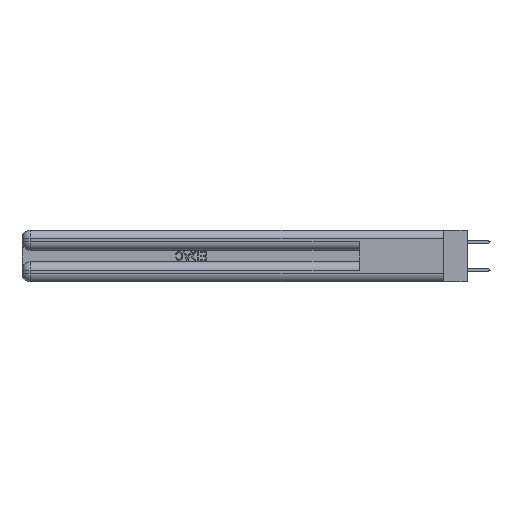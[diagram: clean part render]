
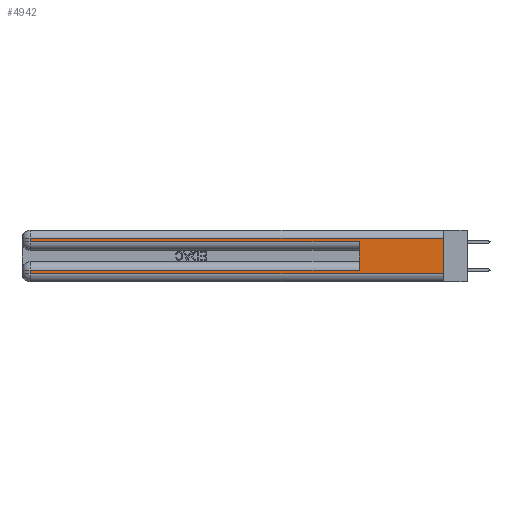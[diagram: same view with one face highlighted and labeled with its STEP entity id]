
A CAD part, left-side view. The second image highlights one B-rep face of the part: STEP entity #4942.
In plain terms, the highlighted planar face has unit normal (-1, 0, 0).
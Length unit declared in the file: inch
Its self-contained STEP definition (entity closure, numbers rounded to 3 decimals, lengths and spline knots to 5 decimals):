
#1281 = LINE ( 'NONE', #5672, #41660 ) ;
#2122 = CARTESIAN_POINT ( 'NONE',  ( 0., 0., 0.06 ) ) ;
#2264 = ORIENTED_EDGE ( 'NONE', *, *, #47043, .T. ) ;
#3876 = EDGE_LOOP ( 'NONE', ( #27338, #7959, #11782, #43535, #30593, #14664, #40190, #2264 ) ) ;
#4942 = ADVANCED_FACE ( 'NONE', ( #32410 ), #41638, .F. ) ;
#4976 = CARTESIAN_POINT ( 'NONE',  ( 0., 0., 0.31 ) ) ;
#5428 = VECTOR ( 'NONE', #43434, 39.37008 ) ;
#5592 = EDGE_CURVE ( 'NONE', #45847, #29594, #26237, .T. ) ;
#5672 = CARTESIAN_POINT ( 'NONE',  ( 0., 0.6, 0.145 ) ) ;
#6160 = DIRECTION ( 'NONE',  ( 0., 0., -1. ) ) ;
#7959 = ORIENTED_EDGE ( 'NONE', *, *, #23020, .T. ) ;
#8643 = VERTEX_POINT ( 'NONE', #48843 ) ;
#8798 = LINE ( 'NONE', #22082, #27135 ) ;
#9466 = DIRECTION ( 'NONE',  ( 0., 0., 1. ) ) ;
#9813 = DIRECTION ( 'NONE',  ( 0., -1., 0. ) ) ;
#11782 = ORIENTED_EDGE ( 'NONE', *, *, #45317, .T. ) ;
#12026 = LINE ( 'NONE', #26265, #30928 ) ;
#14664 = ORIENTED_EDGE ( 'NONE', *, *, #50376, .T. ) ;
#15242 = CARTESIAN_POINT ( 'NONE',  ( 0., 2.94, 0.285 ) ) ;
#16921 = DIRECTION ( 'NONE',  ( 0., 1., 0. ) ) ;
#18801 = EDGE_CURVE ( 'NONE', #29335, #29594, #1281, .T. ) ;
#19373 = VERTEX_POINT ( 'NONE', #39662 ) ;
#19379 = LINE ( 'NONE', #39591, #37740 ) ;
#19396 = DIRECTION ( 'NONE',  ( 0., 0., -1. ) ) ;
#20255 = DIRECTION ( 'NONE',  ( 0., 0., -1. ) ) ;
#21742 = VERTEX_POINT ( 'NONE', #41632 ) ;
#21830 = VECTOR ( 'NONE', #9813, 39.37008 ) ;
#22082 = CARTESIAN_POINT ( 'NONE',  ( 0., 0., 0.37 ) ) ;
#22130 = VERTEX_POINT ( 'NONE', #4976 ) ;
#22729 = CARTESIAN_POINT ( 'NONE',  ( 0., 2.94, 0.37 ) ) ;
#23020 = EDGE_CURVE ( 'NONE', #22130, #42569, #12026, .T. ) ;
#23848 = CARTESIAN_POINT ( 'NONE',  ( 0., 0., 0.37 ) ) ;
#26237 = LINE ( 'NONE', #27685, #5428 ) ;
#26265 = CARTESIAN_POINT ( 'NONE',  ( 0., 0., 0.31 ) ) ;
#26968 = LINE ( 'NONE', #40497, #33716 ) ;
#27076 = DIRECTION ( 'NONE',  ( 1., 0., 0. ) ) ;
#27135 = VECTOR ( 'NONE', #6160, 39.37008 ) ;
#27338 = ORIENTED_EDGE ( 'NONE', *, *, #29759, .F. ) ;
#27685 = CARTESIAN_POINT ( 'NONE',  ( 0., 0., 0.285 ) ) ;
#27855 = LINE ( 'NONE', #22729, #42546 ) ;
#28036 = EDGE_CURVE ( 'NONE', #19373, #21742, #27855, .T. ) ;
#29335 = VERTEX_POINT ( 'NONE', #47261 ) ;
#29594 = VERTEX_POINT ( 'NONE', #44347 ) ;
#29759 = EDGE_CURVE ( 'NONE', #22130, #8643, #8798, .T. ) ;
#30347 = DIRECTION ( 'NONE',  ( 0., 1., 0. ) ) ;
#30593 = ORIENTED_EDGE ( 'NONE', *, *, #18801, .F. ) ;
#30928 = VECTOR ( 'NONE', #30347, 39.37008 ) ;
#32154 = CARTESIAN_POINT ( 'NONE',  ( 0., 2.94, 0.31 ) ) ;
#32410 = FACE_OUTER_BOUND ( 'NONE', #3876, .T. ) ;
#33716 = VECTOR ( 'NONE', #16921, 39.37008 ) ;
#37740 = VECTOR ( 'NONE', #20255, 39.37008 ) ;
#39551 = LINE ( 'NONE', #2122, #21830 ) ;
#39591 = CARTESIAN_POINT ( 'NONE',  ( 0., 2.94, 0.37 ) ) ;
#39662 = CARTESIAN_POINT ( 'NONE',  ( 0., 2.94, 0.085 ) ) ;
#40190 = ORIENTED_EDGE ( 'NONE', *, *, #28036, .T. ) ;
#40497 = CARTESIAN_POINT ( 'NONE',  ( 0., 0., 0.085 ) ) ;
#41632 = CARTESIAN_POINT ( 'NONE',  ( 0., 2.94, 0.06 ) ) ;
#41638 = PLANE ( 'NONE',  #46428 ) ;
#41660 = VECTOR ( 'NONE', #9466, 39.37008 ) ;
#41914 = DIRECTION ( 'NONE',  ( 0., 0., -1. ) ) ;
#42546 = VECTOR ( 'NONE', #41914, 39.37008 ) ;
#42569 = VERTEX_POINT ( 'NONE', #32154 ) ;
#43434 = DIRECTION ( 'NONE',  ( 0., -1., 0. ) ) ;
#43535 = ORIENTED_EDGE ( 'NONE', *, *, #5592, .T. ) ;
#44347 = CARTESIAN_POINT ( 'NONE',  ( 0., 0.6, 0.285 ) ) ;
#45317 = EDGE_CURVE ( 'NONE', #42569, #45847, #19379, .T. ) ;
#45847 = VERTEX_POINT ( 'NONE', #15242 ) ;
#46428 = AXIS2_PLACEMENT_3D ( 'NONE', #23848, #27076, #19396 ) ;
#47043 = EDGE_CURVE ( 'NONE', #21742, #8643, #39551, .T. ) ;
#47261 = CARTESIAN_POINT ( 'NONE',  ( 0., 0.6, 0.085 ) ) ;
#48843 = CARTESIAN_POINT ( 'NONE',  ( 0., 0., 0.06 ) ) ;
#50376 = EDGE_CURVE ( 'NONE', #29335, #19373, #26968, .T. ) ;
